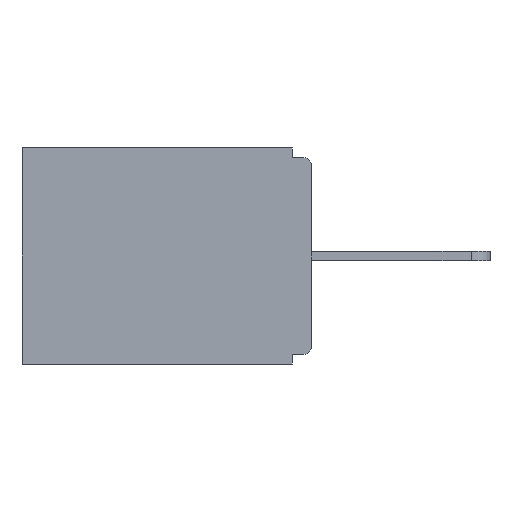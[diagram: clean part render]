
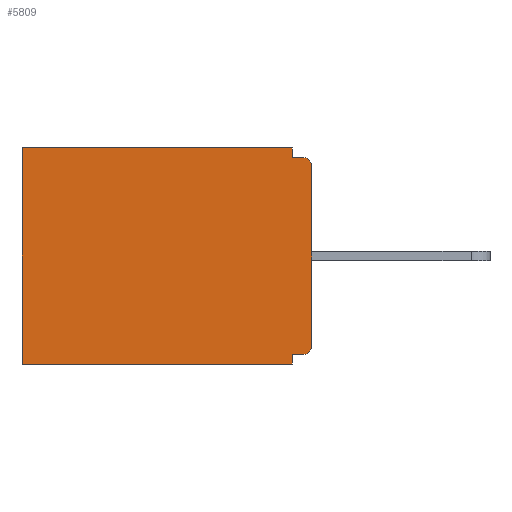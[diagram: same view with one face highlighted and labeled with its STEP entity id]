
A CAD part, left-side view. The second image highlights one B-rep face of the part: STEP entity #5809.
In plain terms, the highlighted planar face has unit normal (-1, 0, 0).
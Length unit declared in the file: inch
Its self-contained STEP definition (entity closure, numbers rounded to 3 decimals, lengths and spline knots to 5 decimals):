
#184 = CARTESIAN_POINT ( 'NONE',  ( 0.298, 0., 0. ) ) ;
#321 = CIRCLE ( 'NONE', #10260, 0.015 ) ;
#334 = ORIENTED_EDGE ( 'NONE', *, *, #1498, .T. ) ;
#358 = ORIENTED_EDGE ( 'NONE', *, *, #4459, .T. ) ;
#368 = DIRECTION ( 'NONE',  ( 0., 1., 0. ) ) ;
#373 = ORIENTED_EDGE ( 'NONE', *, *, #1208, .F. ) ;
#397 = DIRECTION ( 'NONE',  ( 0., -1., 0. ) ) ;
#456 = CARTESIAN_POINT ( 'NONE',  ( 0.298, 0., -0.343 ) ) ;
#622 = DIRECTION ( 'NONE',  ( 0., 0., -1. ) ) ;
#681 = VECTOR ( 'NONE', #9664, 39.37008 ) ;
#724 = CARTESIAN_POINT ( 'NONE',  ( 0.298, 0., -0.313 ) ) ;
#735 = LINE ( 'NONE', #456, #681 ) ;
#894 = EDGE_CURVE ( 'NONE', #6985, #8036, #2969, .T. ) ;
#912 = CARTESIAN_POINT ( 'NONE',  ( 0.298, 0., 0. ) ) ;
#1208 = EDGE_CURVE ( 'NONE', #7184, #3979, #735, .T. ) ;
#1429 = CARTESIAN_POINT ( 'NONE',  ( 0.298, 0., -0.328 ) ) ;
#1498 = EDGE_CURVE ( 'NONE', #7295, #3979, #7282, .T. ) ;
#1629 = EDGE_CURVE ( 'NONE', #8078, #7184, #10603, .T. ) ;
#1963 = CARTESIAN_POINT ( 'NONE',  ( 0.298, 0.015, -0.328 ) ) ;
#2040 = CARTESIAN_POINT ( 'NONE',  ( 0.298, 0.015, -0.015 ) ) ;
#2404 = EDGE_CURVE ( 'NONE', #10718, #8078, #5542, .T. ) ;
#2500 = EDGE_CURVE ( 'NONE', #5306, #6985, #9788, .T. ) ;
#2747 = VECTOR ( 'NONE', #368, 39.37008 ) ;
#2939 = VECTOR ( 'NONE', #397, 39.37008 ) ;
#2969 = LINE ( 'NONE', #5874, #2939 ) ;
#3005 = FACE_OUTER_BOUND ( 'NONE', #9715, .T. ) ;
#3036 = CARTESIAN_POINT ( 'NONE',  ( 0.298, 0.015, -0.03 ) ) ;
#3885 = VECTOR ( 'NONE', #9273, 39.37008 ) ;
#3944 = LINE ( 'NONE', #912, #7874 ) ;
#3964 = CARTESIAN_POINT ( 'NONE',  ( 0.298, 0., -0.03 ) ) ;
#3972 = EDGE_CURVE ( 'NONE', #10625, #4993, #4970, .T. ) ;
#3979 = VERTEX_POINT ( 'NONE', #7911 ) ;
#4131 = VECTOR ( 'NONE', #622, 39.37008 ) ;
#4459 = EDGE_CURVE ( 'NONE', #10718, #4993, #8892, .T. ) ;
#4647 = DIRECTION ( 'NONE',  ( 0., 0., -1. ) ) ;
#4737 = EDGE_CURVE ( 'NONE', #5306, #7295, #3944, .T. ) ;
#4970 = LINE ( 'NONE', #184, #4131 ) ;
#4976 = DIRECTION ( 'NONE',  ( 0., 0., -1. ) ) ;
#4980 = DIRECTION ( 'NONE',  ( 1., 0., 0. ) ) ;
#4993 = VERTEX_POINT ( 'NONE', #724 ) ;
#5270 = ORIENTED_EDGE ( 'NONE', *, *, #3972, .F. ) ;
#5290 = VECTOR ( 'NONE', #10265, 39.37008 ) ;
#5306 = VERTEX_POINT ( 'NONE', #6330 ) ;
#5529 = DIRECTION ( 'NONE',  ( 0., 0., -1. ) ) ;
#5542 = LINE ( 'NONE', #1429, #2747 ) ;
#5809 = ADVANCED_FACE ( 'NONE', ( #3005 ), #8763, .F. ) ;
#5851 = CARTESIAN_POINT ( 'NONE',  ( 0.298, 0.031, -0.343 ) ) ;
#5874 = CARTESIAN_POINT ( 'NONE',  ( 0.298, 0., -0.015 ) ) ;
#6330 = CARTESIAN_POINT ( 'NONE',  ( 0.298, 0.031, 0. ) ) ;
#6434 = CARTESIAN_POINT ( 'NONE',  ( 0.298, 0.46, 0. ) ) ;
#6937 = CARTESIAN_POINT ( 'NONE',  ( 0.298, 0., 0. ) ) ;
#6959 = EDGE_CURVE ( 'NONE', #10625, #8036, #321, .T. ) ;
#6969 = DIRECTION ( 'NONE',  ( 0., 1., 0. ) ) ;
#6985 = VERTEX_POINT ( 'NONE', #7965 ) ;
#7003 = CARTESIAN_POINT ( 'NONE',  ( 0.298, 0.015, -0.313 ) ) ;
#7184 = VERTEX_POINT ( 'NONE', #9645 ) ;
#7282 = LINE ( 'NONE', #6434, #5290 ) ;
#7295 = VERTEX_POINT ( 'NONE', #8947 ) ;
#7367 = AXIS2_PLACEMENT_3D ( 'NONE', #6937, #4980, #4647 ) ;
#7874 = VECTOR ( 'NONE', #6969, 39.37008 ) ;
#7911 = CARTESIAN_POINT ( 'NONE',  ( 0.298, 0.46, -0.343 ) ) ;
#7965 = CARTESIAN_POINT ( 'NONE',  ( 0.298, 0.031, -0.015 ) ) ;
#7978 = DIRECTION ( 'NONE',  ( -1., 0., 0. ) ) ;
#7993 = CARTESIAN_POINT ( 'NONE',  ( 0.298, 0.031, -0.328 ) ) ;
#8036 = VERTEX_POINT ( 'NONE', #2040 ) ;
#8078 = VERTEX_POINT ( 'NONE', #7993 ) ;
#8179 = CARTESIAN_POINT ( 'NONE',  ( 0.298, 0.031, -0.343 ) ) ;
#8475 = DIRECTION ( 'NONE',  ( 0., 0., -1. ) ) ;
#8647 = VECTOR ( 'NONE', #4976, 39.37008 ) ;
#8763 = PLANE ( 'NONE',  #7367 ) ;
#8892 = CIRCLE ( 'NONE', #10442, 0.015 ) ;
#8947 = CARTESIAN_POINT ( 'NONE',  ( 0.298, 0.46, 0. ) ) ;
#9126 = DIRECTION ( 'NONE',  ( -1., 0., 0. ) ) ;
#9273 = DIRECTION ( 'NONE',  ( 0., 0., -1. ) ) ;
#9634 = ORIENTED_EDGE ( 'NONE', *, *, #6959, .T. ) ;
#9645 = CARTESIAN_POINT ( 'NONE',  ( 0.298, 0.031, -0.343 ) ) ;
#9664 = DIRECTION ( 'NONE',  ( 0., 1., 0. ) ) ;
#9715 = EDGE_LOOP ( 'NONE', ( #9634, #9865, #9818, #9959, #334, #373, #10054, #10689, #358, #5270 ) ) ;
#9788 = LINE ( 'NONE', #8179, #3885 ) ;
#9818 = ORIENTED_EDGE ( 'NONE', *, *, #2500, .F. ) ;
#9865 = ORIENTED_EDGE ( 'NONE', *, *, #894, .F. ) ;
#9959 = ORIENTED_EDGE ( 'NONE', *, *, #4737, .T. ) ;
#10054 = ORIENTED_EDGE ( 'NONE', *, *, #1629, .F. ) ;
#10260 = AXIS2_PLACEMENT_3D ( 'NONE', #3036, #9126, #5529 ) ;
#10265 = DIRECTION ( 'NONE',  ( 0., 0., -1. ) ) ;
#10442 = AXIS2_PLACEMENT_3D ( 'NONE', #7003, #7978, #8475 ) ;
#10603 = LINE ( 'NONE', #5851, #8647 ) ;
#10625 = VERTEX_POINT ( 'NONE', #3964 ) ;
#10689 = ORIENTED_EDGE ( 'NONE', *, *, #2404, .F. ) ;
#10718 = VERTEX_POINT ( 'NONE', #1963 ) ;
